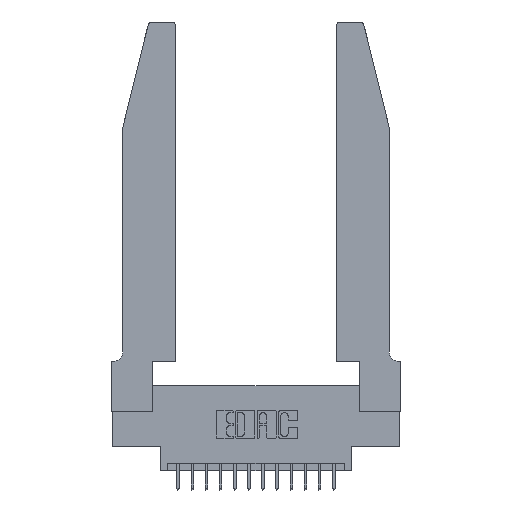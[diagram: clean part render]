
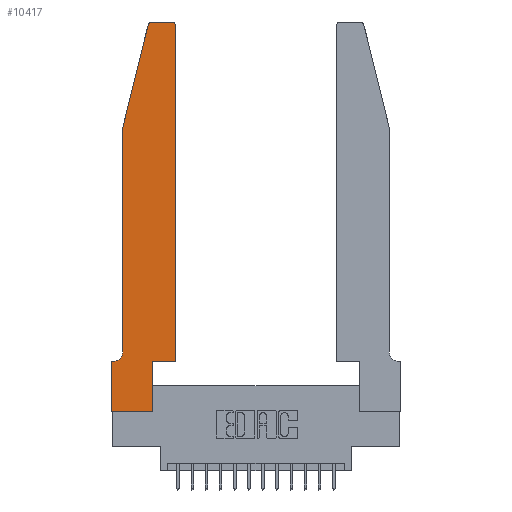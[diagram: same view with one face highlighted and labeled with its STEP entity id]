
A CAD part, top view. The second image highlights one B-rep face of the part: STEP entity #10417.
In plain terms, the highlighted planar face has unit normal (0, 0, 1).
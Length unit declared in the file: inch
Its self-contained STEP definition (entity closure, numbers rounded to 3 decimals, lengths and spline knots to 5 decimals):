
#47 = AXIS2_PLACEMENT_3D ( 'NONE', #18008, #6720, #12414 ) ;
#172 = VECTOR ( 'NONE', #11324, 39.37008 ) ;
#228 = VERTEX_POINT ( 'NONE', #7367 ) ;
#437 = EDGE_CURVE ( 'NONE', #11504, #3470, #16223, .T. ) ;
#533 = CARTESIAN_POINT ( 'NONE',  ( 0.0755, 2., 0.37 ) ) ;
#551 = CARTESIAN_POINT ( 'NONE',  ( 0.284, 2.72, 0.37 ) ) ;
#588 = CARTESIAN_POINT ( 'NONE',  ( 0., 0., 0.37 ) ) ;
#826 = ORIENTED_EDGE ( 'NONE', *, *, #11075, .T. ) ;
#1054 = LINE ( 'NONE', #18045, #13176 ) ;
#1231 = EDGE_CURVE ( 'NONE', #4699, #13682, #1054, .T. ) ;
#1781 = CARTESIAN_POINT ( 'NONE',  ( 0.0755, 0.35, 0.37 ) ) ;
#1842 = CARTESIAN_POINT ( 'NONE',  ( 0.4505, 0.35, 0.37 ) ) ;
#1943 = DIRECTION ( 'NONE',  ( 0., 0., 1. ) ) ;
#2361 = VERTEX_POINT ( 'NONE', #6477 ) ;
#2952 = LINE ( 'NONE', #1842, #5662 ) ;
#2974 = LINE ( 'NONE', #10186, #11580 ) ;
#3244 = VERTEX_POINT ( 'NONE', #6202 ) ;
#3470 = VERTEX_POINT ( 'NONE', #7885 ) ;
#3549 = LINE ( 'NONE', #1781, #11513 ) ;
#3635 = FACE_OUTER_BOUND ( 'NONE', #10087, .T. ) ;
#3942 = DIRECTION ( 'NONE',  ( -1., 0., 0. ) ) ;
#4170 = ORIENTED_EDGE ( 'NONE', *, *, #1231, .T. ) ;
#4236 = ORIENTED_EDGE ( 'NONE', *, *, #17457, .T. ) ;
#4290 = DIRECTION ( 'NONE',  ( 0., 1., 0. ) ) ;
#4547 = VECTOR ( 'NONE', #6233, 39.37008 ) ;
#4699 = VERTEX_POINT ( 'NONE', #17095 ) ;
#4780 = CIRCLE ( 'NONE', #16695, 0.03 ) ;
#4907 = CARTESIAN_POINT ( 'NONE',  ( 0., 0.35, 0.37 ) ) ;
#5162 = DIRECTION ( 'NONE',  ( 0., 0., -1. ) ) ;
#5352 = CARTESIAN_POINT ( 'NONE',  ( 0.0055, 0.42, 0.37 ) ) ;
#5662 = VECTOR ( 'NONE', #17221, 39.37008 ) ;
#5706 = CARTESIAN_POINT ( 'NONE',  ( 0.4505, 2.72, 0.37 ) ) ;
#6202 = CARTESIAN_POINT ( 'NONE',  ( 0.284, 2.75, 0.37 ) ) ;
#6233 = DIRECTION ( 'NONE',  ( -0.239, -0.971, 0. ) ) ;
#6477 = CARTESIAN_POINT ( 'NONE',  ( 0.25487, 2.72718, 0.37 ) ) ;
#6495 = CARTESIAN_POINT ( 'NONE',  ( 0.4205, 2.75, 0.37 ) ) ;
#6720 = DIRECTION ( 'NONE',  ( 0., 0., 1. ) ) ;
#6759 = DIRECTION ( 'NONE',  ( 0., -1., 0. ) ) ;
#7332 = EDGE_CURVE ( 'NONE', #228, #18021, #12602, .T. ) ;
#7367 = CARTESIAN_POINT ( 'NONE',  ( 0.4505, 0.35, 0.37 ) ) ;
#7481 = DIRECTION ( 'NONE',  ( -1., 0., 0. ) ) ;
#7633 = LINE ( 'NONE', #533, #4547 ) ;
#7657 = VECTOR ( 'NONE', #17854, 39.37008 ) ;
#7885 = CARTESIAN_POINT ( 'NONE',  ( 0.2865, 0., 0.37 ) ) ;
#8357 = AXIS2_PLACEMENT_3D ( 'NONE', #17616, #1943, #11847 ) ;
#8482 = ORIENTED_EDGE ( 'NONE', *, *, #9361, .T. ) ;
#8685 = DIRECTION ( 'NONE',  ( 0., 0., 1. ) ) ;
#9142 = CARTESIAN_POINT ( 'NONE',  ( 0.2605, 2.75, 0.37 ) ) ;
#9286 = EDGE_CURVE ( 'NONE', #18021, #17579, #16383, .T. ) ;
#9361 = EDGE_CURVE ( 'NONE', #2361, #4699, #7633, .T. ) ;
#9791 = CARTESIAN_POINT ( 'NONE',  ( 0., 0., 0.37 ) ) ;
#10087 = EDGE_LOOP ( 'NONE', ( #14039, #17980, #8482, #4170, #826, #17743, #12928, #15042, #18047, #4236, #14266, #17448 ) ) ;
#10186 = CARTESIAN_POINT ( 'NONE',  ( 0.2865, 0.35, 0.37 ) ) ;
#10417 = ADVANCED_FACE ( 'NONE', ( #3635 ), #13708, .T. ) ;
#10649 = VERTEX_POINT ( 'NONE', #4907 ) ;
#10832 = AXIS2_PLACEMENT_3D ( 'NONE', #5352, #5162, #3942 ) ;
#10938 = DIRECTION ( 'NONE',  ( 1., 0., 0. ) ) ;
#11075 = EDGE_CURVE ( 'NONE', #13682, #15026, #15859, .T. ) ;
#11324 = DIRECTION ( 'NONE',  ( 0., 1., 0. ) ) ;
#11504 = VERTEX_POINT ( 'NONE', #13797 ) ;
#11513 = VECTOR ( 'NONE', #7481, 39.37008 ) ;
#11580 = VECTOR ( 'NONE', #4290, 39.37008 ) ;
#11673 = VERTEX_POINT ( 'NONE', #12843 ) ;
#11762 = EDGE_CURVE ( 'NONE', #17579, #3244, #14728, .T. ) ;
#11765 = DIRECTION ( 'NONE',  ( -1., 0., 0. ) ) ;
#11847 = DIRECTION ( 'NONE',  ( 1., 0., 0. ) ) ;
#12232 = EDGE_CURVE ( 'NONE', #10649, #11504, #16079, .T. ) ;
#12275 = CARTESIAN_POINT ( 'NONE',  ( 0.0755, 0.42, 0.37 ) ) ;
#12414 = DIRECTION ( 'NONE',  ( 1., 0., 0. ) ) ;
#12602 = LINE ( 'NONE', #13981, #172 ) ;
#12843 = CARTESIAN_POINT ( 'NONE',  ( 0.2865, 0.35, 0.37 ) ) ;
#12844 = EDGE_CURVE ( 'NONE', #15026, #10649, #3549, .T. ) ;
#12928 = ORIENTED_EDGE ( 'NONE', *, *, #12232, .T. ) ;
#13176 = VECTOR ( 'NONE', #6759, 39.37008 ) ;
#13682 = VERTEX_POINT ( 'NONE', #12275 ) ;
#13708 = PLANE ( 'NONE',  #47 ) ;
#13797 = CARTESIAN_POINT ( 'NONE',  ( 0., 0., 0.37 ) ) ;
#13981 = CARTESIAN_POINT ( 'NONE',  ( 0.4505, 0.35, 0.37 ) ) ;
#14039 = ORIENTED_EDGE ( 'NONE', *, *, #11762, .T. ) ;
#14266 = ORIENTED_EDGE ( 'NONE', *, *, #7332, .T. ) ;
#14366 = VECTOR ( 'NONE', #10938, 39.37008 ) ;
#14728 = LINE ( 'NONE', #9142, #16585 ) ;
#15026 = VERTEX_POINT ( 'NONE', #16450 ) ;
#15042 = ORIENTED_EDGE ( 'NONE', *, *, #437, .T. ) ;
#15591 = EDGE_CURVE ( 'NONE', #3470, #11673, #2974, .T. ) ;
#15859 = CIRCLE ( 'NONE', #10832, 0.07 ) ;
#16079 = LINE ( 'NONE', #588, #7657 ) ;
#16223 = LINE ( 'NONE', #9791, #14366 ) ;
#16383 = CIRCLE ( 'NONE', #8357, 0.03 ) ;
#16450 = CARTESIAN_POINT ( 'NONE',  ( 0.0055, 0.35, 0.37 ) ) ;
#16585 = VECTOR ( 'NONE', #11765, 39.37008 ) ;
#16695 = AXIS2_PLACEMENT_3D ( 'NONE', #551, #8685, #17345 ) ;
#17095 = CARTESIAN_POINT ( 'NONE',  ( 0.0755, 2., 0.37 ) ) ;
#17221 = DIRECTION ( 'NONE',  ( 1., 0., 0. ) ) ;
#17345 = DIRECTION ( 'NONE',  ( 1., 0., 0. ) ) ;
#17448 = ORIENTED_EDGE ( 'NONE', *, *, #9286, .T. ) ;
#17457 = EDGE_CURVE ( 'NONE', #11673, #228, #2952, .T. ) ;
#17579 = VERTEX_POINT ( 'NONE', #6495 ) ;
#17616 = CARTESIAN_POINT ( 'NONE',  ( 0.4205, 2.72, 0.37 ) ) ;
#17743 = ORIENTED_EDGE ( 'NONE', *, *, #12844, .T. ) ;
#17854 = DIRECTION ( 'NONE',  ( 0., -1., 0. ) ) ;
#17980 = ORIENTED_EDGE ( 'NONE', *, *, #18135, .T. ) ;
#18008 = CARTESIAN_POINT ( 'NONE',  ( 0., 0.35, 0.37 ) ) ;
#18021 = VERTEX_POINT ( 'NONE', #5706 ) ;
#18045 = CARTESIAN_POINT ( 'NONE',  ( 0.0755, 2., 0.37 ) ) ;
#18047 = ORIENTED_EDGE ( 'NONE', *, *, #15591, .T. ) ;
#18135 = EDGE_CURVE ( 'NONE', #3244, #2361, #4780, .T. ) ;
